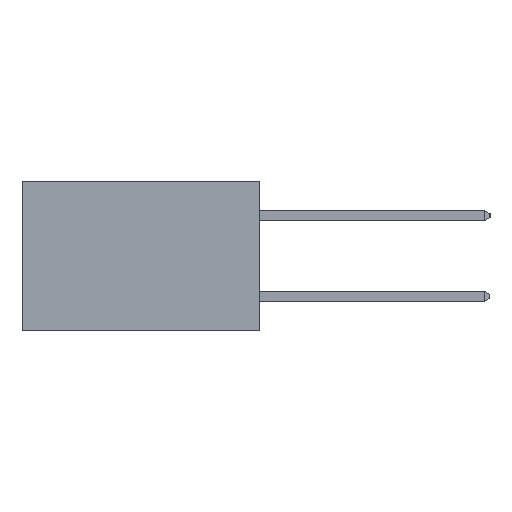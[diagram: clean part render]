
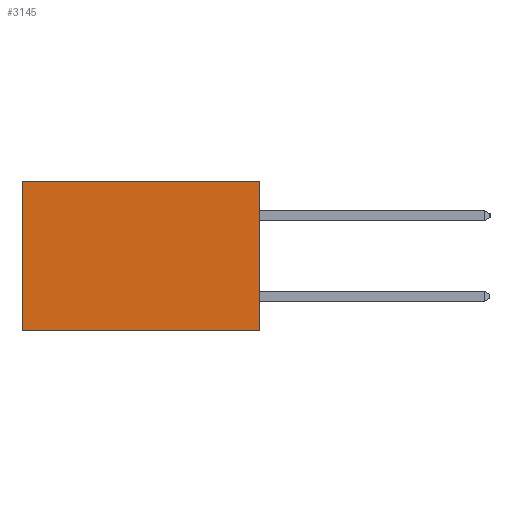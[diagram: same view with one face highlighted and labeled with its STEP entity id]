
A CAD part, left-side view. The second image highlights one B-rep face of the part: STEP entity #3145.
In plain terms, the highlighted planar face has unit normal (-1, 0, 0).
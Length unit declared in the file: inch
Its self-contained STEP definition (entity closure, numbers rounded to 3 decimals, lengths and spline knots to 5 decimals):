
#982 = VECTOR ( 'NONE', #18873, 39.37008 ) ;
#1576 = DIRECTION ( 'NONE',  ( 0., 1., 0. ) ) ;
#1682 = LINE ( 'NONE', #12136, #982 ) ;
#2196 = VERTEX_POINT ( 'NONE', #4777 ) ;
#2556 = LINE ( 'NONE', #5508, #24868 ) ;
#3145 = ADVANCED_FACE ( 'NONE', ( #7245 ), #8784, .F. ) ;
#3210 = DIRECTION ( 'NONE',  ( 0., 0., -1. ) ) ;
#3285 = EDGE_LOOP ( 'NONE', ( #21928, #23726, #22553, #13822 ) ) ;
#4777 = CARTESIAN_POINT ( 'NONE',  ( 0.277, 0.59, 0. ) ) ;
#5028 = EDGE_CURVE ( 'NONE', #6094, #25545, #2556, .T. ) ;
#5508 = CARTESIAN_POINT ( 'NONE',  ( 0.277, 0., -0.37 ) ) ;
#6094 = VERTEX_POINT ( 'NONE', #22438 ) ;
#7245 = FACE_OUTER_BOUND ( 'NONE', #3285, .T. ) ;
#8784 = PLANE ( 'NONE',  #11000 ) ;
#9790 = CARTESIAN_POINT ( 'NONE',  ( 0.277, 0., -0.37 ) ) ;
#10377 = EDGE_CURVE ( 'NONE', #18967, #6094, #19512, .T. ) ;
#11000 = AXIS2_PLACEMENT_3D ( 'NONE', #18228, #16789, #20858 ) ;
#11156 = EDGE_CURVE ( 'NONE', #2196, #25545, #15607, .T. ) ;
#12136 = CARTESIAN_POINT ( 'NONE',  ( 0.277, 0., 0. ) ) ;
#13822 = ORIENTED_EDGE ( 'NONE', *, *, #19481, .T. ) ;
#15607 = LINE ( 'NONE', #24892, #26763 ) ;
#16769 = CARTESIAN_POINT ( 'NONE',  ( 0.277, 0.59, -0.37 ) ) ;
#16789 = DIRECTION ( 'NONE',  ( 1., 0., 0. ) ) ;
#17128 = CARTESIAN_POINT ( 'NONE',  ( 0.277, 0., 0. ) ) ;
#18228 = CARTESIAN_POINT ( 'NONE',  ( 0.277, 0., -0.37 ) ) ;
#18873 = DIRECTION ( 'NONE',  ( 0., 1., 0. ) ) ;
#18967 = VERTEX_POINT ( 'NONE', #17128 ) ;
#19481 = EDGE_CURVE ( 'NONE', #18967, #2196, #1682, .T. ) ;
#19512 = LINE ( 'NONE', #9790, #24779 ) ;
#20858 = DIRECTION ( 'NONE',  ( 0., 0., -1. ) ) ;
#21928 = ORIENTED_EDGE ( 'NONE', *, *, #11156, .T. ) ;
#22438 = CARTESIAN_POINT ( 'NONE',  ( 0.277, 0., -0.37 ) ) ;
#22553 = ORIENTED_EDGE ( 'NONE', *, *, #10377, .F. ) ;
#23726 = ORIENTED_EDGE ( 'NONE', *, *, #5028, .F. ) ;
#24779 = VECTOR ( 'NONE', #3210, 39.37008 ) ;
#24868 = VECTOR ( 'NONE', #1576, 39.37008 ) ;
#24892 = CARTESIAN_POINT ( 'NONE',  ( 0.277, 0.59, -0.37 ) ) ;
#25545 = VERTEX_POINT ( 'NONE', #16769 ) ;
#26763 = VECTOR ( 'NONE', #27063, 39.37008 ) ;
#27063 = DIRECTION ( 'NONE',  ( 0., 0., -1. ) ) ;
